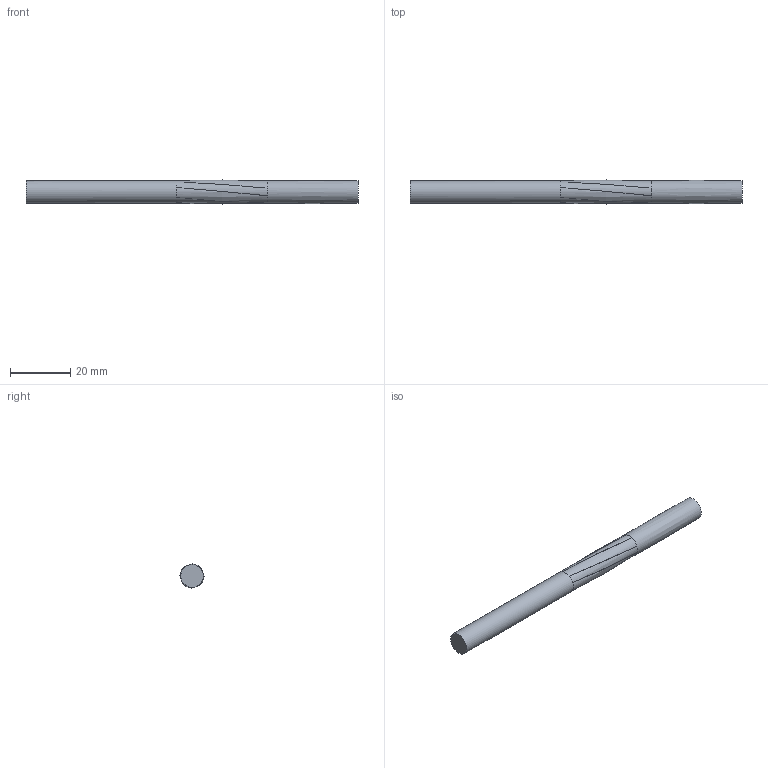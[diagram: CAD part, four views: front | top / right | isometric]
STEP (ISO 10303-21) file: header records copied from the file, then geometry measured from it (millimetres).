
FILE_DESCRIPTION(/* description */ (''),/* implementation_level */ '2;1');
FILE_NAME(/* name */ '.308 rifling button.stp',/* time_stamp */ '2020-12-13T23:05:33+09:00',/* author */ ('user'),/* organization */ (''),/* preprocessor_version */ 'ST-DEVELOPER v16.5',/* originating_system */ 'Autodesk Inventor 2017',/* authorisation */ '');
FILE_SCHEMA (('AUTOMOTIVE_DESIGN { 1 0 10303 214 3 1 1 }'));
Length unit declared in the file: inch
Products named in the file (1): Part2
Bounding box: 110 x 7.96 x 7.96 mm (x, y, z)
Volume: 4959 mm3; surface area: 2757.5 mm2
Topology: 1 solids, 1 shells, 20 faces, 39 edges, 21 vertices
Faces by surface type: bspline 13, cylinder 5, plane 2
Full cylindrical faces by diameter (mm): 7.5 x1
Entity records: 910 total; most frequent: CARTESIAN_POINT 546, ORIENTED_EDGE 74, DIRECTION 56, EDGE_CURVE 37, AXIS2_PLACEMENT_3D 28, EDGE_LOOP 21, FACE_OUTER_BOUND 20, CIRCLE 20
